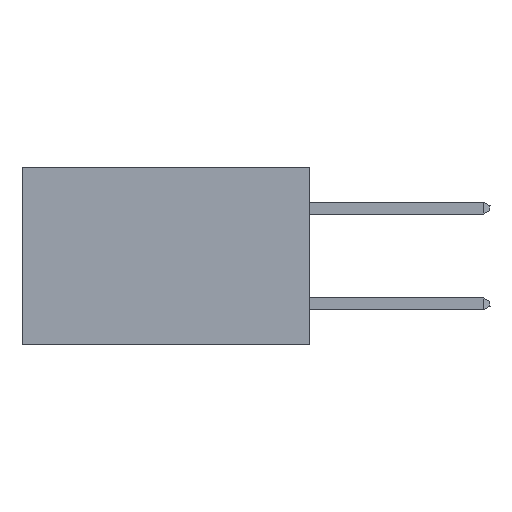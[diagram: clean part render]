
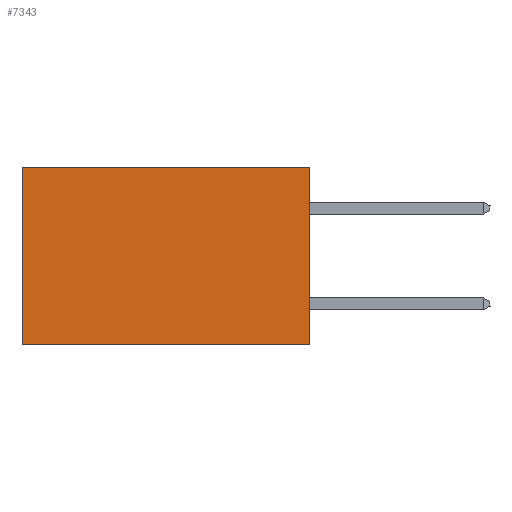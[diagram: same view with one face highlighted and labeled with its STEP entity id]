
A CAD part, left-side view. The second image highlights one B-rep face of the part: STEP entity #7343.
In plain terms, the highlighted planar face has unit normal (-1, 0, 0).
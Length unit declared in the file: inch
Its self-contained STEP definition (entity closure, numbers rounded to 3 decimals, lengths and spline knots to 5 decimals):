
#1703 = EDGE_CURVE ( 'NONE', #23288, #8034, #13705, .T. ) ;
#2229 = DIRECTION ( 'NONE',  ( 0., 0., -1. ) ) ;
#2563 = ORIENTED_EDGE ( 'NONE', *, *, #1703, .F. ) ;
#4295 = DIRECTION ( 'NONE',  ( 0., 0., -1. ) ) ;
#6174 = CARTESIAN_POINT ( 'NONE',  ( 0.2875, 0., 0. ) ) ;
#7343 = ADVANCED_FACE ( 'NONE', ( #14727 ), #22592, .F. ) ;
#7535 = CARTESIAN_POINT ( 'NONE',  ( 0.2875, 0., -0.37 ) ) ;
#8034 = VERTEX_POINT ( 'NONE', #7535 ) ;
#8264 = ORIENTED_EDGE ( 'NONE', *, *, #24898, .T. ) ;
#9209 = VECTOR ( 'NONE', #27302, 39.37008 ) ;
#9633 = LINE ( 'NONE', #6174, #12123 ) ;
#9658 = EDGE_CURVE ( 'NONE', #23608, #14090, #17801, .T. ) ;
#10013 = CARTESIAN_POINT ( 'NONE',  ( 0.2875, 0.6, 0. ) ) ;
#10369 = VECTOR ( 'NONE', #14462, 39.37008 ) ;
#11378 = CARTESIAN_POINT ( 'NONE',  ( 0.2875, 0.6, 0. ) ) ;
#12123 = VECTOR ( 'NONE', #13018, 39.37008 ) ;
#12449 = CARTESIAN_POINT ( 'NONE',  ( 0.2875, 0., -0.37 ) ) ;
#13018 = DIRECTION ( 'NONE',  ( 0., 1., 0. ) ) ;
#13657 = EDGE_CURVE ( 'NONE', #8034, #14090, #16457, .T. ) ;
#13705 = LINE ( 'NONE', #15652, #22601 ) ;
#14090 = VERTEX_POINT ( 'NONE', #19599 ) ;
#14462 = DIRECTION ( 'NONE',  ( 0., 1., 0. ) ) ;
#14727 = FACE_OUTER_BOUND ( 'NONE', #23386, .T. ) ;
#15119 = CARTESIAN_POINT ( 'NONE',  ( 0.2875, 0., 0. ) ) ;
#15648 = CARTESIAN_POINT ( 'NONE',  ( 0.2875, 0., 0. ) ) ;
#15652 = CARTESIAN_POINT ( 'NONE',  ( 0.2875, 0., 0. ) ) ;
#15858 = DIRECTION ( 'NONE',  ( 1., 0., 0. ) ) ;
#16457 = LINE ( 'NONE', #12449, #10369 ) ;
#17449 = ORIENTED_EDGE ( 'NONE', *, *, #9658, .T. ) ;
#17801 = LINE ( 'NONE', #11378, #9209 ) ;
#18406 = AXIS2_PLACEMENT_3D ( 'NONE', #15648, #15858, #2229 ) ;
#19599 = CARTESIAN_POINT ( 'NONE',  ( 0.2875, 0.6, -0.37 ) ) ;
#22592 = PLANE ( 'NONE',  #18406 ) ;
#22601 = VECTOR ( 'NONE', #4295, 39.37008 ) ;
#23288 = VERTEX_POINT ( 'NONE', #15119 ) ;
#23386 = EDGE_LOOP ( 'NONE', ( #17449, #27023, #2563, #8264 ) ) ;
#23608 = VERTEX_POINT ( 'NONE', #10013 ) ;
#24898 = EDGE_CURVE ( 'NONE', #23288, #23608, #9633, .T. ) ;
#27023 = ORIENTED_EDGE ( 'NONE', *, *, #13657, .F. ) ;
#27302 = DIRECTION ( 'NONE',  ( 0., 0., -1. ) ) ;
